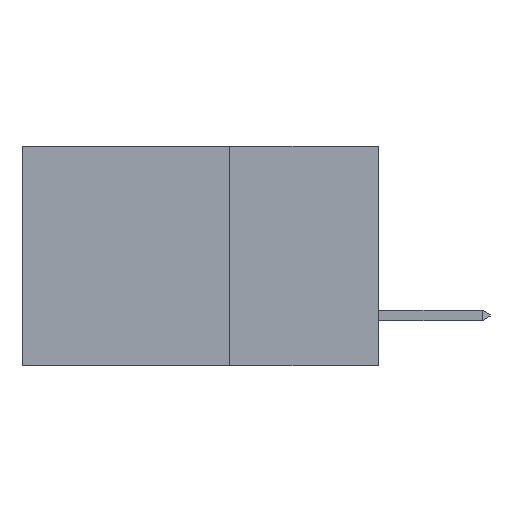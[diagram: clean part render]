
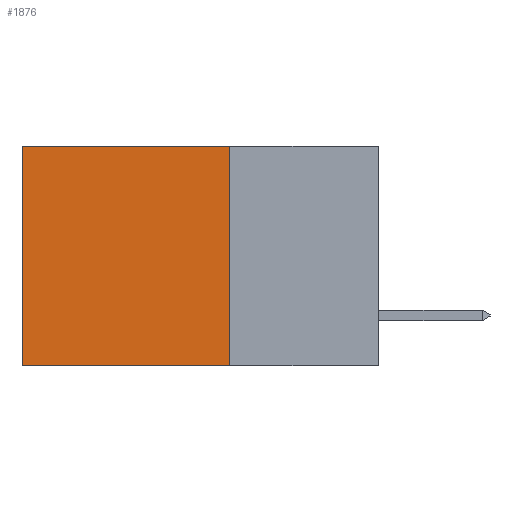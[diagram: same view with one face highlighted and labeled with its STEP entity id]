
A CAD part, left-side view. The second image highlights one B-rep face of the part: STEP entity #1876.
In plain terms, the highlighted planar face has unit normal (-1, 0, 0).
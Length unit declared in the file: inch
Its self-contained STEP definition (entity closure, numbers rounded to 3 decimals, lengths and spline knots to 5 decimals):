
#293 = CARTESIAN_POINT ( 'NONE',  ( 0.2615, 0.25, -0.37 ) ) ;
#1876 = ADVANCED_FACE ( 'NONE', ( #9927 ), #14582, .F. ) ;
#1893 = VERTEX_POINT ( 'NONE', #12045 ) ;
#2204 = ORIENTED_EDGE ( 'NONE', *, *, #18656, .T. ) ;
#2834 = CARTESIAN_POINT ( 'NONE',  ( 0.2615, 0.6, 0. ) ) ;
#4518 = VECTOR ( 'NONE', #14977, 39.37008 ) ;
#5686 = CARTESIAN_POINT ( 'NONE',  ( 0.2615, 0.25, 0. ) ) ;
#5978 = EDGE_CURVE ( 'NONE', #1893, #14199, #21569, .T. ) ;
#6176 = DIRECTION ( 'NONE',  ( 0., 0., -1. ) ) ;
#7469 = VECTOR ( 'NONE', #19913, 39.37008 ) ;
#7778 = CARTESIAN_POINT ( 'NONE',  ( 0.2615, 0.25, -0.37 ) ) ;
#9927 = FACE_OUTER_BOUND ( 'NONE', #19665, .T. ) ;
#10619 = LINE ( 'NONE', #7778, #19421 ) ;
#10986 = ORIENTED_EDGE ( 'NONE', *, *, #5978, .T. ) ;
#11405 = VECTOR ( 'NONE', #6176, 39.37008 ) ;
#12045 = CARTESIAN_POINT ( 'NONE',  ( 0.2615, 0.25, 0. ) ) ;
#12937 = DIRECTION ( 'NONE',  ( 0., 0., -1. ) ) ;
#13072 = DIRECTION ( 'NONE',  ( 1., 0., 0. ) ) ;
#13243 = CARTESIAN_POINT ( 'NONE',  ( 0.2615, 0.25, -0.37 ) ) ;
#13708 = CARTESIAN_POINT ( 'NONE',  ( 0.2615, 0.25, -0.37 ) ) ;
#14047 = EDGE_CURVE ( 'NONE', #1893, #15251, #14674, .T. ) ;
#14199 = VERTEX_POINT ( 'NONE', #2834 ) ;
#14582 = PLANE ( 'NONE',  #14615 ) ;
#14615 = AXIS2_PLACEMENT_3D ( 'NONE', #13708, #13072, #12937 ) ;
#14674 = LINE ( 'NONE', #13243, #4518 ) ;
#14977 = DIRECTION ( 'NONE',  ( 0., 0., -1. ) ) ;
#15098 = CARTESIAN_POINT ( 'NONE',  ( 0.2615, 0.6, -0.37 ) ) ;
#15251 = VERTEX_POINT ( 'NONE', #293 ) ;
#16073 = LINE ( 'NONE', #15098, #11405 ) ;
#17883 = VERTEX_POINT ( 'NONE', #20240 ) ;
#18656 = EDGE_CURVE ( 'NONE', #14199, #17883, #16073, .T. ) ;
#19421 = VECTOR ( 'NONE', #21900, 39.37008 ) ;
#19665 = EDGE_LOOP ( 'NONE', ( #2204, #21688, #20501, #10986 ) ) ;
#19913 = DIRECTION ( 'NONE',  ( 0., 1., 0. ) ) ;
#20240 = CARTESIAN_POINT ( 'NONE',  ( 0.2615, 0.6, -0.37 ) ) ;
#20501 = ORIENTED_EDGE ( 'NONE', *, *, #14047, .F. ) ;
#21569 = LINE ( 'NONE', #5686, #7469 ) ;
#21688 = ORIENTED_EDGE ( 'NONE', *, *, #22683, .F. ) ;
#21900 = DIRECTION ( 'NONE',  ( 0., 1., 0. ) ) ;
#22683 = EDGE_CURVE ( 'NONE', #15251, #17883, #10619, .T. ) ;
